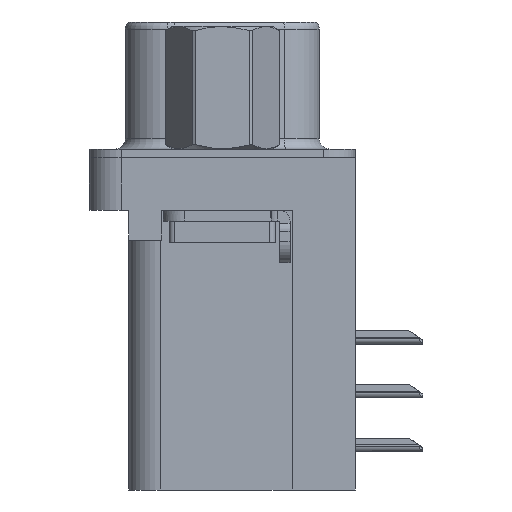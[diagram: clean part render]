
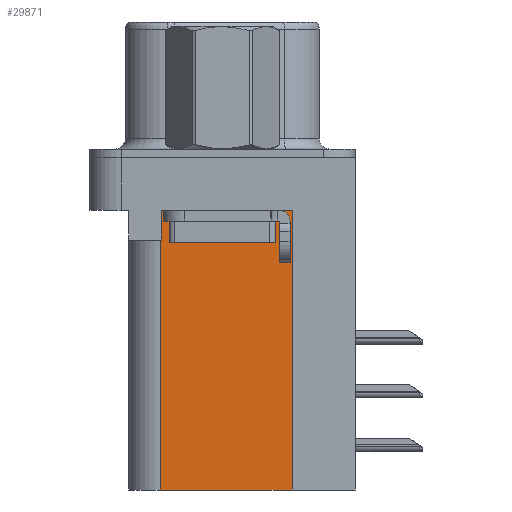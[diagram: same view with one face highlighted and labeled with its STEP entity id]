
A CAD part, left-side view. The second image highlights one B-rep face of the part: STEP entity #29871.
In plain terms, the highlighted planar face has unit normal (-1, 0, 0).
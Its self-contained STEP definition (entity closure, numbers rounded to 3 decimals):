
#497 = ORIENTED_EDGE ( 'NONE', *, *, #34942, .T. ) ;
#907 = VERTEX_POINT ( 'NONE', #25459 ) ;
#1118 = CARTESIAN_POINT ( 'NONE',  ( 3.79, 2.895, -2.5 ) ) ;
#1389 = VECTOR ( 'NONE', #18582, 1000. ) ;
#2314 = CARTESIAN_POINT ( 'NONE',  ( 3.79, 2.895, -3.9 ) ) ;
#5351 = DIRECTION ( 'NONE',  ( 0., 0., -1. ) ) ;
#5571 = DIRECTION ( 'NONE',  ( 0., 0., 1. ) ) ;
#6213 = CARTESIAN_POINT ( 'NONE',  ( 3.79, 2.925, -3.9 ) ) ;
#6707 = LINE ( 'NONE', #20302, #38309 ) ;
#7212 = PLANE ( 'NONE',  #34992 ) ;
#7408 = VERTEX_POINT ( 'NONE', #36553 ) ;
#8462 = LINE ( 'NONE', #19900, #31745 ) ;
#8622 = ORIENTED_EDGE ( 'NONE', *, *, #14802, .F. ) ;
#10809 = CARTESIAN_POINT ( 'NONE',  ( 3.79, 2.895, -3.9 ) ) ;
#11456 = LINE ( 'NONE', #2314, #34956 ) ;
#13027 = FACE_OUTER_BOUND ( 'NONE', #32198, .T. ) ;
#13197 = DIRECTION ( 'NONE',  ( 0., 0., -1. ) ) ;
#14403 = DIRECTION ( 'NONE',  ( 0., 1., 0. ) ) ;
#14501 = VECTOR ( 'NONE', #5571, 1000. ) ;
#14802 = EDGE_CURVE ( 'NONE', #7408, #907, #25348, .T. ) ;
#15499 = EDGE_CURVE ( 'NONE', #7408, #18718, #8462, .T. ) ;
#16595 = ORIENTED_EDGE ( 'NONE', *, *, #15499, .T. ) ;
#17410 = VERTEX_POINT ( 'NONE', #6213 ) ;
#18582 = DIRECTION ( 'NONE',  ( 0., 1., 0. ) ) ;
#18718 = VERTEX_POINT ( 'NONE', #36330 ) ;
#19900 = CARTESIAN_POINT ( 'NONE',  ( 3.79, -3.295, -15.7 ) ) ;
#20302 = CARTESIAN_POINT ( 'NONE',  ( 3.79, 0., -3.9 ) ) ;
#20430 = CARTESIAN_POINT ( 'NONE',  ( 3.79, 2.925, -15.7 ) ) ;
#21589 = CARTESIAN_POINT ( 'NONE',  ( 3.79, -3.295, -15.7 ) ) ;
#23148 = DIRECTION ( 'NONE',  ( 0., 1., 0. ) ) ;
#23412 = LINE ( 'NONE', #20430, #14501 ) ;
#25348 = LINE ( 'NONE', #21589, #1389 ) ;
#25459 = CARTESIAN_POINT ( 'NONE',  ( 3.79, 2.925, -15.7 ) ) ;
#25991 = DIRECTION ( 'NONE',  ( 0., 0., 1. ) ) ;
#27103 = ORIENTED_EDGE ( 'NONE', *, *, #36701, .T. ) ;
#27451 = ORIENTED_EDGE ( 'NONE', *, *, #38321, .F. ) ;
#28293 = CARTESIAN_POINT ( 'NONE',  ( 3.79, -3.295, -15.7 ) ) ;
#29871 = ADVANCED_FACE ( 'NONE', ( #13027 ), #7212, .F. ) ;
#30283 = VERTEX_POINT ( 'NONE', #10809 ) ;
#31514 = DIRECTION ( 'NONE',  ( 1., 0., 0. ) ) ;
#31745 = VECTOR ( 'NONE', #25991, 1000. ) ;
#32198 = EDGE_LOOP ( 'NONE', ( #33519, #497, #27103, #27451, #8622, #16595 ) ) ;
#33519 = ORIENTED_EDGE ( 'NONE', *, *, #33949, .T. ) ;
#33949 = EDGE_CURVE ( 'NONE', #18718, #34256, #36540, .T. ) ;
#34256 = VERTEX_POINT ( 'NONE', #1118 ) ;
#34942 = EDGE_CURVE ( 'NONE', #34256, #30283, #11456, .T. ) ;
#34956 = VECTOR ( 'NONE', #5351, 1000. ) ;
#34992 = AXIS2_PLACEMENT_3D ( 'NONE', #28293, #31514, #13197 ) ;
#35565 = VECTOR ( 'NONE', #23148, 1000. ) ;
#36330 = CARTESIAN_POINT ( 'NONE',  ( 3.79, -3.295, -2.5 ) ) ;
#36540 = LINE ( 'NONE', #38811, #35565 ) ;
#36553 = CARTESIAN_POINT ( 'NONE',  ( 3.79, -3.295, -15.7 ) ) ;
#36701 = EDGE_CURVE ( 'NONE', #30283, #17410, #6707, .T. ) ;
#38309 = VECTOR ( 'NONE', #14403, 1000. ) ;
#38321 = EDGE_CURVE ( 'NONE', #907, #17410, #23412, .T. ) ;
#38811 = CARTESIAN_POINT ( 'NONE',  ( 3.79, -3.295, -2.5 ) ) ;
